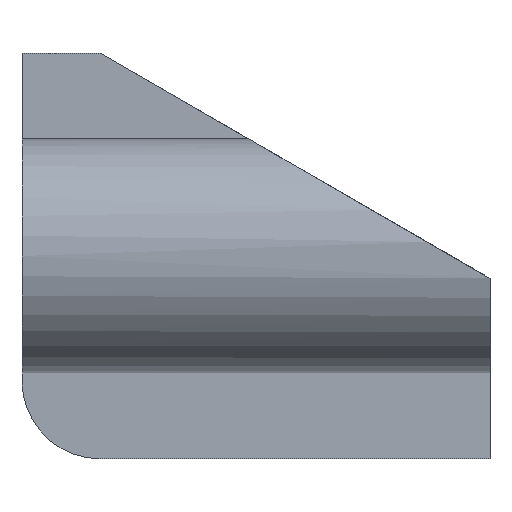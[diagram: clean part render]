
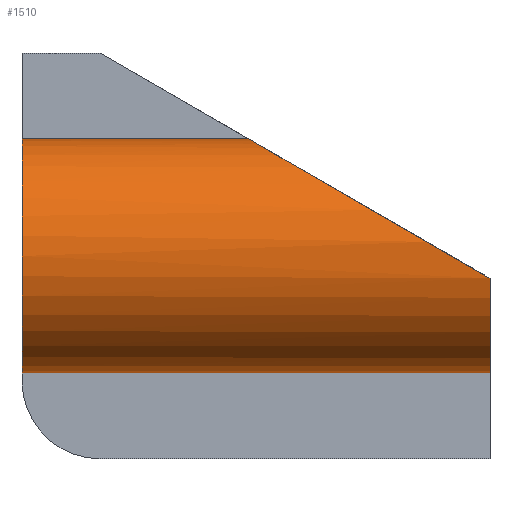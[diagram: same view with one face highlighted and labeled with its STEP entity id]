
A CAD part, front view. The second image highlights one B-rep face of the part: STEP entity #1510.
In plain terms, the highlighted cylindrical face has radius 9.525 mm (diameter 19.05 mm), a partial arc.
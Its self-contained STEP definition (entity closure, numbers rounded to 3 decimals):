
#157 = PLANE('',#158);
#158 = AXIS2_PLACEMENT_3D('',#159,#160,#161);
#159 = CARTESIAN_POINT('',(19.05,21.996,14.689));
#160 = DIRECTION('',(-0.5,0.,-0.866));
#161 = DIRECTION('',(-0.866,0.,0.5));
#350 = PLANE('',#351);
#351 = AXIS2_PLACEMENT_3D('',#352,#353,#354);
#352 = CARTESIAN_POINT('',(19.05,0.,0.));
#353 = DIRECTION('',(0.,-1.,0.));
#354 = DIRECTION('',(-1.,0.,0.));
#501 = VERTEX_POINT('',#502);
#502 = CARTESIAN_POINT('',(19.05,0.,6.985));
#516 = PLANE('',#517);
#517 = AXIS2_PLACEMENT_3D('',#518,#519,#520);
#518 = CARTESIAN_POINT('',(19.05,0.,26.035));
#519 = DIRECTION('',(-1.,0.,0.));
#520 = DIRECTION('',(0.,0.,-1.));
#555 = VERTEX_POINT('',#556);
#556 = CARTESIAN_POINT('',(-19.05,0.,6.985));
#578 = VERTEX_POINT('',#579);
#579 = CARTESIAN_POINT('',(-19.05,0.,26.035));
#593 = PLANE('',#594);
#594 = AXIS2_PLACEMENT_3D('',#595,#596,#597);
#595 = CARTESIAN_POINT('',(-19.05,0.,0.));
#596 = DIRECTION('',(-1.,0.,0.));
#597 = DIRECTION('',(-0.,-1.,-0.));
#620 = PLANE('',#621);
#621 = AXIS2_PLACEMENT_3D('',#622,#623,#624);
#622 = CARTESIAN_POINT('',(19.05,0.,0.));
#623 = DIRECTION('',(0.,-1.,0.));
#624 = DIRECTION('',(-1.,0.,0.));
#851 = VERTEX_POINT('',#852);
#852 = CARTESIAN_POINT('',(19.05,-9.349,14.689));
#873 = EDGE_CURVE('',#851,#874,#876,.T.);
#874 = VERTEX_POINT('',#875);
#875 = CARTESIAN_POINT('',(-0.602,0.,26.035));
#876 = SURFACE_CURVE('',#877,(#882,#889),.PCURVE_S1.);
#877 = ELLIPSE('',#878,19.05,9.525);
#878 = AXIS2_PLACEMENT_3D('',#879,#880,#881);
#879 = CARTESIAN_POINT('',(15.896,0.,16.51));
#880 = DIRECTION('',(-0.5,0.,-0.866));
#881 = DIRECTION('',(0.866,0.,-0.5));
#882 = PCURVE('',#157,#883);
#883 = DEFINITIONAL_REPRESENTATION('',(#884),#888);
#884 = ELLIPSE('',#885,19.05,9.525);
#885 = AXIS2_PLACEMENT_2D('',#886,#887);
#886 = CARTESIAN_POINT('',(3.642,-21.996));
#887 = DIRECTION('',(-1.,0.));
#888 = ( GEOMETRIC_REPRESENTATION_CONTEXT(2) 
PARAMETRIC_REPRESENTATION_CONTEXT() REPRESENTATION_CONTEXT('2D SPACE',''
  ) );
#889 = PCURVE('',#890,#895);
#890 = CYLINDRICAL_SURFACE('',#891,9.525);
#891 = AXIS2_PLACEMENT_3D('',#892,#893,#894);
#892 = CARTESIAN_POINT('',(19.05,0.,16.51));
#893 = DIRECTION('',(1.,0.,0.));
#894 = DIRECTION('',(0.,1.,0.));
#895 = DEFINITIONAL_REPRESENTATION('',(#896),#907);
#896 = B_SPLINE_CURVE_WITH_KNOTS('',9,(#897,#898,#899,#900,#901,#902,
    #903,#904,#905,#906),.UNSPECIFIED.,.F.,.F.,(10,10),(1.378,
    3.142),.PIECEWISE_BEZIER_KNOTS.);
#897 = CARTESIAN_POINT('',(3.334,0.));
#898 = CARTESIAN_POINT('',(3.138,-3.172));
#899 = CARTESIAN_POINT('',(2.942,-6.481));
#900 = CARTESIAN_POINT('',(2.746,-9.75));
#901 = CARTESIAN_POINT('',(2.55,-12.792));
#902 = CARTESIAN_POINT('',(2.354,-15.43));
#903 = CARTESIAN_POINT('',(2.159,-17.515));
#904 = CARTESIAN_POINT('',(1.963,-18.939));
#905 = CARTESIAN_POINT('',(1.767,-19.652));
#906 = CARTESIAN_POINT('',(1.571,-19.652));
#907 = ( GEOMETRIC_REPRESENTATION_CONTEXT(2) 
PARAMETRIC_REPRESENTATION_CONTEXT() REPRESENTATION_CONTEXT('2D SPACE',''
  ) );
#1100 = EDGE_CURVE('',#501,#555,#1101,.T.);
#1101 = SURFACE_CURVE('',#1102,(#1106,#1113),.PCURVE_S1.);
#1102 = LINE('',#1103,#1104);
#1103 = CARTESIAN_POINT('',(19.05,0.,6.985));
#1104 = VECTOR('',#1105,1.);
#1105 = DIRECTION('',(-1.,-0.,-0.));
#1106 = PCURVE('',#350,#1107);
#1107 = DEFINITIONAL_REPRESENTATION('',(#1108),#1112);
#1108 = LINE('',#1109,#1110);
#1109 = CARTESIAN_POINT('',(0.,-6.985));
#1110 = VECTOR('',#1111,1.);
#1111 = DIRECTION('',(1.,0.));
#1112 = ( GEOMETRIC_REPRESENTATION_CONTEXT(2) 
PARAMETRIC_REPRESENTATION_CONTEXT() REPRESENTATION_CONTEXT('2D SPACE',''
  ) );
#1113 = PCURVE('',#890,#1114);
#1114 = DEFINITIONAL_REPRESENTATION('',(#1115),#1119);
#1115 = LINE('',#1116,#1117);
#1116 = CARTESIAN_POINT('',(4.712,0.));
#1117 = VECTOR('',#1118,1.);
#1118 = DIRECTION('',(0.,-1.));
#1119 = ( GEOMETRIC_REPRESENTATION_CONTEXT(2) 
PARAMETRIC_REPRESENTATION_CONTEXT() REPRESENTATION_CONTEXT('2D SPACE',''
  ) );
#1342 = EDGE_CURVE('',#851,#501,#1343,.T.);
#1343 = SURFACE_CURVE('',#1344,(#1349,#1360),.PCURVE_S1.);
#1344 = CIRCLE('',#1345,9.525);
#1345 = AXIS2_PLACEMENT_3D('',#1346,#1347,#1348);
#1346 = CARTESIAN_POINT('',(19.05,0.,16.51));
#1347 = DIRECTION('',(1.,0.,0.));
#1348 = DIRECTION('',(0.,1.,0.));
#1349 = PCURVE('',#516,#1350);
#1350 = DEFINITIONAL_REPRESENTATION('',(#1351),#1359);
#1351 = ( BOUNDED_CURVE() B_SPLINE_CURVE(2,(#1352,#1353,#1354,#1355,
#1356,#1357,#1358),.UNSPECIFIED.,.F.,.F.) B_SPLINE_CURVE_WITH_KNOTS((1,2
    ,2,2,2,1),(-2.094,0.,2.094,4.189,
6.283,8.378),.UNSPECIFIED.) CURVE() 
GEOMETRIC_REPRESENTATION_ITEM() RATIONAL_B_SPLINE_CURVE((1.,0.5,1.,0.5,
1.,0.5,1.)) REPRESENTATION_ITEM('') );
#1352 = CARTESIAN_POINT('',(9.525,-9.525));
#1353 = CARTESIAN_POINT('',(-6.973,-9.525));
#1354 = CARTESIAN_POINT('',(1.276,4.763));
#1355 = CARTESIAN_POINT('',(9.525,19.05));
#1356 = CARTESIAN_POINT('',(17.774,4.763));
#1357 = CARTESIAN_POINT('',(26.023,-9.525));
#1358 = CARTESIAN_POINT('',(9.525,-9.525));
#1359 = ( GEOMETRIC_REPRESENTATION_CONTEXT(2) 
PARAMETRIC_REPRESENTATION_CONTEXT() REPRESENTATION_CONTEXT('2D SPACE',''
  ) );
#1360 = PCURVE('',#890,#1361);
#1361 = DEFINITIONAL_REPRESENTATION('',(#1362),#1366);
#1362 = LINE('',#1363,#1364);
#1363 = CARTESIAN_POINT('',(0.,0.));
#1364 = VECTOR('',#1365,1.);
#1365 = DIRECTION('',(1.,0.));
#1366 = ( GEOMETRIC_REPRESENTATION_CONTEXT(2) 
PARAMETRIC_REPRESENTATION_CONTEXT() REPRESENTATION_CONTEXT('2D SPACE',''
  ) );
#1400 = EDGE_CURVE('',#578,#555,#1401,.T.);
#1401 = SURFACE_CURVE('',#1402,(#1407,#1418),.PCURVE_S1.);
#1402 = CIRCLE('',#1403,9.525);
#1403 = AXIS2_PLACEMENT_3D('',#1404,#1405,#1406);
#1404 = CARTESIAN_POINT('',(-19.05,0.,16.51));
#1405 = DIRECTION('',(1.,0.,0.));
#1406 = DIRECTION('',(0.,1.,0.));
#1407 = PCURVE('',#593,#1408);
#1408 = DEFINITIONAL_REPRESENTATION('',(#1409),#1417);
#1409 = ( BOUNDED_CURVE() B_SPLINE_CURVE(2,(#1410,#1411,#1412,#1413,
#1414,#1415,#1416),.UNSPECIFIED.,.T.,.F.) B_SPLINE_CURVE_WITH_KNOTS((1,2
    ,2,2,2,1),(-2.094,0.,2.094,4.189,
6.283,8.378),.UNSPECIFIED.) CURVE() 
GEOMETRIC_REPRESENTATION_ITEM() RATIONAL_B_SPLINE_CURVE((1.,0.5,1.,0.5,
1.,0.5,1.)) REPRESENTATION_ITEM('') );
#1410 = CARTESIAN_POINT('',(-9.525,16.51));
#1411 = CARTESIAN_POINT('',(-9.525,33.008));
#1412 = CARTESIAN_POINT('',(4.763,24.759));
#1413 = CARTESIAN_POINT('',(19.05,16.51));
#1414 = CARTESIAN_POINT('',(4.763,8.261));
#1415 = CARTESIAN_POINT('',(-9.525,0.012));
#1416 = CARTESIAN_POINT('',(-9.525,16.51));
#1417 = ( GEOMETRIC_REPRESENTATION_CONTEXT(2) 
PARAMETRIC_REPRESENTATION_CONTEXT() REPRESENTATION_CONTEXT('2D SPACE',''
  ) );
#1418 = PCURVE('',#890,#1419);
#1419 = DEFINITIONAL_REPRESENTATION('',(#1420),#1424);
#1420 = LINE('',#1421,#1422);
#1421 = CARTESIAN_POINT('',(0.,-38.1));
#1422 = VECTOR('',#1423,1.);
#1423 = DIRECTION('',(1.,0.));
#1424 = ( GEOMETRIC_REPRESENTATION_CONTEXT(2) 
PARAMETRIC_REPRESENTATION_CONTEXT() REPRESENTATION_CONTEXT('2D SPACE',''
  ) );
#1460 = EDGE_CURVE('',#874,#578,#1461,.T.);
#1461 = SURFACE_CURVE('',#1462,(#1466,#1473),.PCURVE_S1.);
#1462 = LINE('',#1463,#1464);
#1463 = CARTESIAN_POINT('',(19.05,0.,26.035));
#1464 = VECTOR('',#1465,1.);
#1465 = DIRECTION('',(-1.,-0.,-0.));
#1466 = PCURVE('',#620,#1467);
#1467 = DEFINITIONAL_REPRESENTATION('',(#1468),#1472);
#1468 = LINE('',#1469,#1470);
#1469 = CARTESIAN_POINT('',(0.,-26.035));
#1470 = VECTOR('',#1471,1.);
#1471 = DIRECTION('',(1.,0.));
#1472 = ( GEOMETRIC_REPRESENTATION_CONTEXT(2) 
PARAMETRIC_REPRESENTATION_CONTEXT() REPRESENTATION_CONTEXT('2D SPACE',''
  ) );
#1473 = PCURVE('',#890,#1474);
#1474 = DEFINITIONAL_REPRESENTATION('',(#1475),#1479);
#1475 = LINE('',#1476,#1477);
#1476 = CARTESIAN_POINT('',(1.571,0.));
#1477 = VECTOR('',#1478,1.);
#1478 = DIRECTION('',(0.,-1.));
#1479 = ( GEOMETRIC_REPRESENTATION_CONTEXT(2) 
PARAMETRIC_REPRESENTATION_CONTEXT() REPRESENTATION_CONTEXT('2D SPACE',''
  ) );
#1510 = ADVANCED_FACE('',(#1511),#890,.T.);
#1511 = FACE_BOUND('',#1512,.T.);
#1512 = EDGE_LOOP('',(#1513,#1514,#1515,#1516,#1517));
#1513 = ORIENTED_EDGE('',*,*,#1342,.F.);
#1514 = ORIENTED_EDGE('',*,*,#873,.T.);
#1515 = ORIENTED_EDGE('',*,*,#1460,.T.);
#1516 = ORIENTED_EDGE('',*,*,#1400,.T.);
#1517 = ORIENTED_EDGE('',*,*,#1100,.F.);
